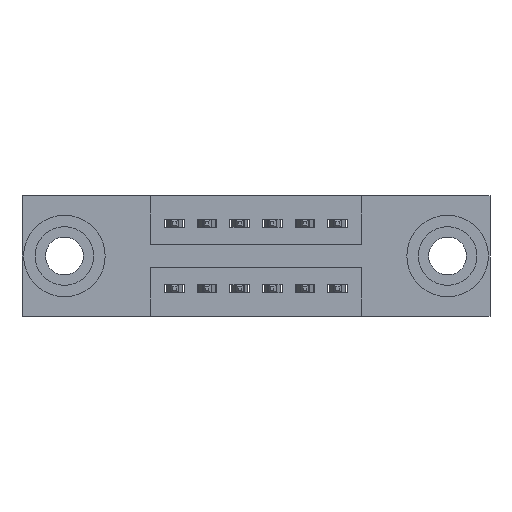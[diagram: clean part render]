
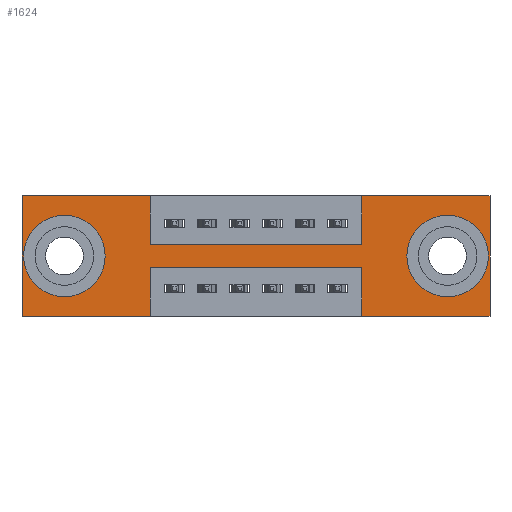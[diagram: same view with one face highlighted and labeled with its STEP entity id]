
A CAD part, front view. The second image highlights one B-rep face of the part: STEP entity #1624.
In plain terms, the highlighted planar face has unit normal (0, -1, 0).
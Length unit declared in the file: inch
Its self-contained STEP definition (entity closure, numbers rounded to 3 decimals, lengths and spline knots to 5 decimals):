
#61 = CIRCLE ( 'NONE', #7061, 0.078 ) ;
#113 = DIRECTION ( 'NONE',  ( 0., -1., 0. ) ) ;
#158 = AXIS2_PLACEMENT_3D ( 'NONE', #9386, #6190, #7732 ) ;
#162 = ORIENTED_EDGE ( 'NONE', *, *, #8731, .T. ) ;
#167 = CARTESIAN_POINT ( 'NONE',  ( 1.305, 0., -0.185 ) ) ;
#319 = CARTESIAN_POINT ( 'NONE',  ( 1.435, 0., -0.37 ) ) ;
#456 = VECTOR ( 'NONE', #5387, 39.37008 ) ;
#520 = CARTESIAN_POINT ( 'NONE',  ( 1.435, 0., 0. ) ) ;
#523 = CARTESIAN_POINT ( 'NONE',  ( 0.3925, 0., -0.15 ) ) ;
#812 = VERTEX_POINT ( 'NONE', #4695 ) ;
#899 = VERTEX_POINT ( 'NONE', #2466 ) ;
#960 = CARTESIAN_POINT ( 'NONE',  ( 0.13, 0., -0.263 ) ) ;
#988 = FACE_BOUND ( 'NONE', #5001, .T. ) ;
#1030 = CARTESIAN_POINT ( 'NONE',  ( 0., 0., -0.37 ) ) ;
#1151 = EDGE_CURVE ( 'NONE', #9480, #899, #9012, .T. ) ;
#1201 = LINE ( 'NONE', #6955, #3593 ) ;
#1290 = CARTESIAN_POINT ( 'NONE',  ( 0., 0., 0. ) ) ;
#1365 = VERTEX_POINT ( 'NONE', #7373 ) ;
#1479 = LINE ( 'NONE', #4553, #1719 ) ;
#1582 = CARTESIAN_POINT ( 'NONE',  ( 0.13, 0., -0.185 ) ) ;
#1624 = ADVANCED_FACE ( 'NONE', ( #6310, #988, #8031 ), #7763, .T. ) ;
#1692 = VERTEX_POINT ( 'NONE', #319 ) ;
#1719 = VECTOR ( 'NONE', #4677, 39.37008 ) ;
#1723 = ORIENTED_EDGE ( 'NONE', *, *, #4390, .T. ) ;
#1809 = EDGE_CURVE ( 'NONE', #1365, #10097, #2626, .T. ) ;
#1849 = ORIENTED_EDGE ( 'NONE', *, *, #3059, .F. ) ;
#2094 = AXIS2_PLACEMENT_3D ( 'NONE', #1582, #10084, #5423 ) ;
#2123 = VERTEX_POINT ( 'NONE', #5598 ) ;
#2133 = CARTESIAN_POINT ( 'NONE',  ( 0.3925, 0., -0.37 ) ) ;
#2407 = VERTEX_POINT ( 'NONE', #960 ) ;
#2430 = EDGE_CURVE ( 'NONE', #1692, #812, #3358, .T. ) ;
#2466 = CARTESIAN_POINT ( 'NONE',  ( 1.435, 0., 0. ) ) ;
#2529 = DIRECTION ( 'NONE',  ( 0., 1., 0. ) ) ;
#2626 = LINE ( 'NONE', #6307, #5576 ) ;
#2633 = LINE ( 'NONE', #7594, #4713 ) ;
#2671 = DIRECTION ( 'NONE',  ( 0., 0., 1. ) ) ;
#2740 = ORIENTED_EDGE ( 'NONE', *, *, #4871, .F. ) ;
#2774 = ORIENTED_EDGE ( 'NONE', *, *, #7186, .F. ) ;
#2854 = DIRECTION ( 'NONE',  ( 0., 0., -1. ) ) ;
#2863 = ORIENTED_EDGE ( 'NONE', *, *, #3992, .F. ) ;
#2957 = ORIENTED_EDGE ( 'NONE', *, *, #9263, .T. ) ;
#3018 = CARTESIAN_POINT ( 'NONE',  ( 1.305, 0., -0.107 ) ) ;
#3059 = EDGE_CURVE ( 'NONE', #7927, #8215, #1201, .T. ) ;
#3114 = VERTEX_POINT ( 'NONE', #7840 ) ;
#3225 = CARTESIAN_POINT ( 'NONE',  ( 1.305, 0., -0.185 ) ) ;
#3358 = LINE ( 'NONE', #1030, #4582 ) ;
#3503 = CARTESIAN_POINT ( 'NONE',  ( 1.0425, 0., -0.37 ) ) ;
#3530 = ORIENTED_EDGE ( 'NONE', *, *, #1809, .F. ) ;
#3558 = DIRECTION ( 'NONE',  ( 1., 0., 0. ) ) ;
#3593 = VECTOR ( 'NONE', #8462, 39.37008 ) ;
#3694 = EDGE_CURVE ( 'NONE', #812, #7927, #6385, .T. ) ;
#3750 = EDGE_CURVE ( 'NONE', #899, #1692, #8716, .T. ) ;
#3819 = CARTESIAN_POINT ( 'NONE',  ( 0., 0., -0.37 ) ) ;
#3959 = VERTEX_POINT ( 'NONE', #5268 ) ;
#3992 = EDGE_CURVE ( 'NONE', #8215, #10101, #6374, .T. ) ;
#4066 = ORIENTED_EDGE ( 'NONE', *, *, #8592, .T. ) ;
#4099 = ORIENTED_EDGE ( 'NONE', *, *, #7970, .F. ) ;
#4158 = DIRECTION ( 'NONE',  ( 0., 0., -1. ) ) ;
#4178 = CARTESIAN_POINT ( 'NONE',  ( 1.0425, 0., 0. ) ) ;
#4390 = EDGE_CURVE ( 'NONE', #6845, #2407, #5746, .T. ) ;
#4528 = CARTESIAN_POINT ( 'NONE',  ( 0., 0., -0.37 ) ) ;
#4553 = CARTESIAN_POINT ( 'NONE',  ( 0.3925, 0., 0. ) ) ;
#4582 = VECTOR ( 'NONE', #8890, 39.37008 ) ;
#4621 = DIRECTION ( 'NONE',  ( 0., 0., -1. ) ) ;
#4677 = DIRECTION ( 'NONE',  ( 0., 0., -1. ) ) ;
#4679 = DIRECTION ( 'NONE',  ( 1., 0., 0. ) ) ;
#4695 = CARTESIAN_POINT ( 'NONE',  ( 1.0425, 0., -0.37 ) ) ;
#4713 = VECTOR ( 'NONE', #10102, 39.37008 ) ;
#4767 = DIRECTION ( 'NONE',  ( 0., 0., 1. ) ) ;
#4769 = ORIENTED_EDGE ( 'NONE', *, *, #2430, .F. ) ;
#4871 = EDGE_CURVE ( 'NONE', #10097, #3114, #6859, .T. ) ;
#5000 = ORIENTED_EDGE ( 'NONE', *, *, #3694, .F. ) ;
#5001 = EDGE_LOOP ( 'NONE', ( #1723, #2957 ) ) ;
#5025 = VECTOR ( 'NONE', #3558, 39.37008 ) ;
#5268 = CARTESIAN_POINT ( 'NONE',  ( 1.0425, 0., -0.15 ) ) ;
#5305 = EDGE_LOOP ( 'NONE', ( #162, #4066 ) ) ;
#5387 = DIRECTION ( 'NONE',  ( -1., 0., 0. ) ) ;
#5405 = DIRECTION ( 'NONE',  ( 1., 0., 0. ) ) ;
#5423 = DIRECTION ( 'NONE',  ( 0., 0., 1. ) ) ;
#5534 = VECTOR ( 'NONE', #2854, 39.37008 ) ;
#5576 = VECTOR ( 'NONE', #4767, 39.37008 ) ;
#5598 = CARTESIAN_POINT ( 'NONE',  ( 1.305, 0., -0.263 ) ) ;
#5615 = AXIS2_PLACEMENT_3D ( 'NONE', #167, #2529, #4158 ) ;
#5646 = VECTOR ( 'NONE', #2671, 39.37008 ) ;
#5746 = CIRCLE ( 'NONE', #2094, 0.078 ) ;
#6005 = VECTOR ( 'NONE', #4621, 39.37008 ) ;
#6034 = CARTESIAN_POINT ( 'NONE',  ( 0., 0., 0. ) ) ;
#6190 = DIRECTION ( 'NONE',  ( 0., 1., 0. ) ) ;
#6198 = VERTEX_POINT ( 'NONE', #7019 ) ;
#6307 = CARTESIAN_POINT ( 'NONE',  ( 0., 0., 0. ) ) ;
#6310 = FACE_BOUND ( 'NONE', #5305, .T. ) ;
#6374 = LINE ( 'NONE', #7683, #6005 ) ;
#6385 = LINE ( 'NONE', #3503, #5646 ) ;
#6473 = AXIS2_PLACEMENT_3D ( 'NONE', #4528, #113, #6666 ) ;
#6577 = CARTESIAN_POINT ( 'NONE',  ( 0.13, 0., -0.107 ) ) ;
#6666 = DIRECTION ( 'NONE',  ( 0., 0., -1. ) ) ;
#6845 = VERTEX_POINT ( 'NONE', #6577 ) ;
#6859 = LINE ( 'NONE', #6034, #5025 ) ;
#6955 = CARTESIAN_POINT ( 'NONE',  ( 0.3925, 0., -0.22 ) ) ;
#7019 = CARTESIAN_POINT ( 'NONE',  ( 0.3925, 0., -0.15 ) ) ;
#7061 = AXIS2_PLACEMENT_3D ( 'NONE', #3225, #9520, #9487 ) ;
#7186 = EDGE_CURVE ( 'NONE', #6198, #3959, #7891, .T. ) ;
#7243 = EDGE_CURVE ( 'NONE', #3959, #9480, #2633, .T. ) ;
#7373 = CARTESIAN_POINT ( 'NONE',  ( 0., 0., -0.37 ) ) ;
#7594 = CARTESIAN_POINT ( 'NONE',  ( 1.0425, 0., 0. ) ) ;
#7683 = CARTESIAN_POINT ( 'NONE',  ( 0.3925, 0., -0.37 ) ) ;
#7732 = DIRECTION ( 'NONE',  ( 0., 0., 1. ) ) ;
#7763 = PLANE ( 'NONE',  #6473 ) ;
#7794 = CARTESIAN_POINT ( 'NONE',  ( 0., 0., 0. ) ) ;
#7840 = CARTESIAN_POINT ( 'NONE',  ( 0.3925, 0., 0. ) ) ;
#7891 = LINE ( 'NONE', #523, #9990 ) ;
#7927 = VERTEX_POINT ( 'NONE', #9265 ) ;
#7970 = EDGE_CURVE ( 'NONE', #3114, #6198, #1479, .T. ) ;
#7999 = VERTEX_POINT ( 'NONE', #3018 ) ;
#8031 = FACE_OUTER_BOUND ( 'NONE', #8180, .T. ) ;
#8116 = ORIENTED_EDGE ( 'NONE', *, *, #1151, .F. ) ;
#8180 = EDGE_LOOP ( 'NONE', ( #2863, #1849, #5000, #4769, #9171, #8116, #8701, #2774, #4099, #2740, #3530, #9674 ) ) ;
#8215 = VERTEX_POINT ( 'NONE', #9627 ) ;
#8357 = CIRCLE ( 'NONE', #158, 0.078 ) ;
#8462 = DIRECTION ( 'NONE',  ( -1., 0., 0. ) ) ;
#8470 = EDGE_CURVE ( 'NONE', #10101, #1365, #9957, .T. ) ;
#8592 = EDGE_CURVE ( 'NONE', #2123, #7999, #61, .T. ) ;
#8701 = ORIENTED_EDGE ( 'NONE', *, *, #7243, .F. ) ;
#8716 = LINE ( 'NONE', #520, #5534 ) ;
#8731 = EDGE_CURVE ( 'NONE', #7999, #2123, #9697, .T. ) ;
#8890 = DIRECTION ( 'NONE',  ( -1., 0., 0. ) ) ;
#8896 = VECTOR ( 'NONE', #4679, 39.37008 ) ;
#9012 = LINE ( 'NONE', #7794, #8896 ) ;
#9171 = ORIENTED_EDGE ( 'NONE', *, *, #3750, .F. ) ;
#9263 = EDGE_CURVE ( 'NONE', #2407, #6845, #8357, .T. ) ;
#9265 = CARTESIAN_POINT ( 'NONE',  ( 1.0425, 0., -0.22 ) ) ;
#9386 = CARTESIAN_POINT ( 'NONE',  ( 0.13, 0., -0.185 ) ) ;
#9480 = VERTEX_POINT ( 'NONE', #4178 ) ;
#9487 = DIRECTION ( 'NONE',  ( 0., 0., -1. ) ) ;
#9520 = DIRECTION ( 'NONE',  ( 0., 1., 0. ) ) ;
#9627 = CARTESIAN_POINT ( 'NONE',  ( 0.3925, 0., -0.22 ) ) ;
#9674 = ORIENTED_EDGE ( 'NONE', *, *, #8470, .F. ) ;
#9697 = CIRCLE ( 'NONE', #5615, 0.078 ) ;
#9957 = LINE ( 'NONE', #3819, #456 ) ;
#9990 = VECTOR ( 'NONE', #5405, 39.37008 ) ;
#10084 = DIRECTION ( 'NONE',  ( 0., 1., 0. ) ) ;
#10097 = VERTEX_POINT ( 'NONE', #1290 ) ;
#10101 = VERTEX_POINT ( 'NONE', #2133 ) ;
#10102 = DIRECTION ( 'NONE',  ( 0., 0., 1. ) ) ;
